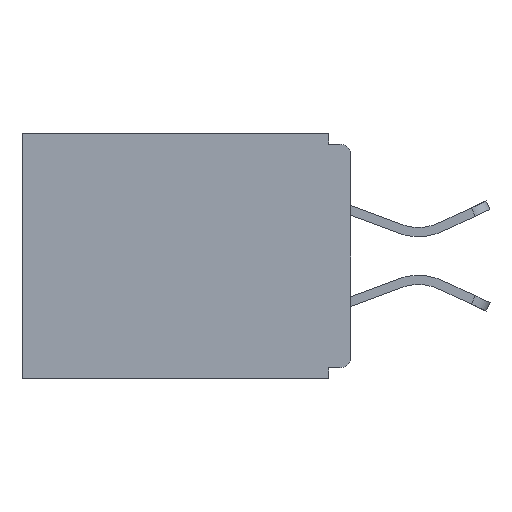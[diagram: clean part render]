
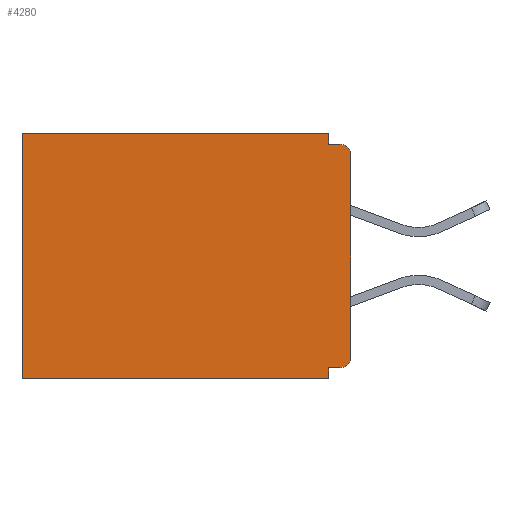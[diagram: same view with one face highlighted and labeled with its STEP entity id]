
A CAD part, left-side view. The second image highlights one B-rep face of the part: STEP entity #4280.
In plain terms, the highlighted planar face has unit normal (-1, 0, 0).
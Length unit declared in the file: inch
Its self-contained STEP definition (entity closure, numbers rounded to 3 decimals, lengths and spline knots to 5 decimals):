
#148 = DIRECTION ( 'NONE',  ( 0., 0., -1. ) ) ;
#595 = DIRECTION ( 'NONE',  ( -1., 0., 0. ) ) ;
#615 = PLANE ( 'NONE',  #6951 ) ;
#616 = VERTEX_POINT ( 'NONE', #11996 ) ;
#864 = VERTEX_POINT ( 'NONE', #12964 ) ;
#898 = CARTESIAN_POINT ( 'NONE',  ( 0.298, 0.031, -0.015 ) ) ;
#1536 = VERTEX_POINT ( 'NONE', #4678 ) ;
#1597 = EDGE_CURVE ( 'NONE', #10476, #2965, #2961, .T. ) ;
#1646 = CARTESIAN_POINT ( 'NONE',  ( 0.298, 0.031, -0.343 ) ) ;
#1675 = VERTEX_POINT ( 'NONE', #11287 ) ;
#1849 = CARTESIAN_POINT ( 'NONE',  ( 0.298, 0., 0. ) ) ;
#1911 = EDGE_CURVE ( 'NONE', #1536, #12967, #3587, .T. ) ;
#1960 = LINE ( 'NONE', #8977, #10019 ) ;
#1978 = VECTOR ( 'NONE', #6179, 39.37008 ) ;
#2581 = CARTESIAN_POINT ( 'NONE',  ( 0.298, 0.031, -0.343 ) ) ;
#2738 = CARTESIAN_POINT ( 'NONE',  ( 0.298, 0.015, -0.03 ) ) ;
#2759 = DIRECTION ( 'NONE',  ( 1., 0., 0. ) ) ;
#2955 = EDGE_CURVE ( 'NONE', #12348, #10156, #1960, .T. ) ;
#2961 = LINE ( 'NONE', #2581, #11042 ) ;
#2965 = VERTEX_POINT ( 'NONE', #1646 ) ;
#3064 = DIRECTION ( 'NONE',  ( 0., 1., 0. ) ) ;
#3109 = VECTOR ( 'NONE', #12346, 39.37008 ) ;
#3587 = LINE ( 'NONE', #12476, #8893 ) ;
#3760 = ORIENTED_EDGE ( 'NONE', *, *, #2955, .F. ) ;
#3929 = DIRECTION ( 'NONE',  ( 0., 0., -1. ) ) ;
#3978 = CARTESIAN_POINT ( 'NONE',  ( 0.298, 0.015, -0.015 ) ) ;
#4077 = ORIENTED_EDGE ( 'NONE', *, *, #9372, .T. ) ;
#4238 = ORIENTED_EDGE ( 'NONE', *, *, #1597, .F. ) ;
#4280 = ADVANCED_FACE ( 'NONE', ( #4674 ), #615, .F. ) ;
#4674 = FACE_OUTER_BOUND ( 'NONE', #10426, .T. ) ;
#4678 = CARTESIAN_POINT ( 'NONE',  ( 0.298, 0.031, 0. ) ) ;
#4708 = AXIS2_PLACEMENT_3D ( 'NONE', #8175, #6306, #9445 ) ;
#5553 = DIRECTION ( 'NONE',  ( 0., -1., 0. ) ) ;
#5603 = ORIENTED_EDGE ( 'NONE', *, *, #7041, .F. ) ;
#5711 = ORIENTED_EDGE ( 'NONE', *, *, #7684, .F. ) ;
#6006 = VERTEX_POINT ( 'NONE', #11267 ) ;
#6042 = ORIENTED_EDGE ( 'NONE', *, *, #1911, .T. ) ;
#6179 = DIRECTION ( 'NONE',  ( 0., 0., -1. ) ) ;
#6188 = DIRECTION ( 'NONE',  ( 0., 1., 0. ) ) ;
#6306 = DIRECTION ( 'NONE',  ( -1., 0., 0. ) ) ;
#6473 = ORIENTED_EDGE ( 'NONE', *, *, #11056, .T. ) ;
#6628 = VECTOR ( 'NONE', #8684, 39.37008 ) ;
#6683 = VECTOR ( 'NONE', #148, 39.37008 ) ;
#6951 = AXIS2_PLACEMENT_3D ( 'NONE', #1849, #2759, #3929 ) ;
#7041 = EDGE_CURVE ( 'NONE', #2965, #864, #10455, .T. ) ;
#7437 = CARTESIAN_POINT ( 'NONE',  ( 0.298, 0., 0. ) ) ;
#7562 = ORIENTED_EDGE ( 'NONE', *, *, #8576, .T. ) ;
#7569 = LINE ( 'NONE', #13562, #1978 ) ;
#7634 = VECTOR ( 'NONE', #3064, 39.37008 ) ;
#7684 = EDGE_CURVE ( 'NONE', #1675, #6006, #8781, .T. ) ;
#7711 = CARTESIAN_POINT ( 'NONE',  ( 0.298, 0.46, 0. ) ) ;
#7928 = DIRECTION ( 'NONE',  ( 0., 0., -1. ) ) ;
#7967 = AXIS2_PLACEMENT_3D ( 'NONE', #2738, #595, #7928 ) ;
#8098 = CARTESIAN_POINT ( 'NONE',  ( 0.298, 0., -0.328 ) ) ;
#8175 = CARTESIAN_POINT ( 'NONE',  ( 0.298, 0.015, -0.313 ) ) ;
#8576 = EDGE_CURVE ( 'NONE', #1675, #10156, #9905, .T. ) ;
#8684 = DIRECTION ( 'NONE',  ( 0., 0., -1. ) ) ;
#8781 = LINE ( 'NONE', #7437, #6628 ) ;
#8893 = VECTOR ( 'NONE', #6188, 39.37008 ) ;
#8977 = CARTESIAN_POINT ( 'NONE',  ( 0.298, 0., -0.015 ) ) ;
#9044 = EDGE_CURVE ( 'NONE', #616, #10476, #12858, .T. ) ;
#9372 = EDGE_CURVE ( 'NONE', #12967, #864, #7569, .T. ) ;
#9445 = DIRECTION ( 'NONE',  ( 0., 0., -1. ) ) ;
#9905 = CIRCLE ( 'NONE', #7967, 0.015 ) ;
#10019 = VECTOR ( 'NONE', #5553, 39.37008 ) ;
#10156 = VERTEX_POINT ( 'NONE', #3978 ) ;
#10426 = EDGE_LOOP ( 'NONE', ( #7562, #3760, #10877, #6042, #4077, #5603, #4238, #11911, #6473, #5711 ) ) ;
#10455 = LINE ( 'NONE', #11515, #7634 ) ;
#10476 = VERTEX_POINT ( 'NONE', #10955 ) ;
#10877 = ORIENTED_EDGE ( 'NONE', *, *, #11201, .F. ) ;
#10955 = CARTESIAN_POINT ( 'NONE',  ( 0.298, 0.031, -0.328 ) ) ;
#10969 = CIRCLE ( 'NONE', #4708, 0.015 ) ;
#11042 = VECTOR ( 'NONE', #12104, 39.37008 ) ;
#11056 = EDGE_CURVE ( 'NONE', #616, #6006, #10969, .T. ) ;
#11201 = EDGE_CURVE ( 'NONE', #1536, #12348, #12635, .T. ) ;
#11267 = CARTESIAN_POINT ( 'NONE',  ( 0.298, 0., -0.313 ) ) ;
#11287 = CARTESIAN_POINT ( 'NONE',  ( 0.298, 0., -0.03 ) ) ;
#11515 = CARTESIAN_POINT ( 'NONE',  ( 0.298, 0., -0.343 ) ) ;
#11846 = CARTESIAN_POINT ( 'NONE',  ( 0.298, 0.031, -0.343 ) ) ;
#11911 = ORIENTED_EDGE ( 'NONE', *, *, #9044, .F. ) ;
#11996 = CARTESIAN_POINT ( 'NONE',  ( 0.298, 0.015, -0.328 ) ) ;
#12104 = DIRECTION ( 'NONE',  ( 0., 0., -1. ) ) ;
#12346 = DIRECTION ( 'NONE',  ( 0., 1., 0. ) ) ;
#12348 = VERTEX_POINT ( 'NONE', #898 ) ;
#12476 = CARTESIAN_POINT ( 'NONE',  ( 0.298, 0., 0. ) ) ;
#12635 = LINE ( 'NONE', #11846, #6683 ) ;
#12858 = LINE ( 'NONE', #8098, #3109 ) ;
#12964 = CARTESIAN_POINT ( 'NONE',  ( 0.298, 0.46, -0.343 ) ) ;
#12967 = VERTEX_POINT ( 'NONE', #7711 ) ;
#13562 = CARTESIAN_POINT ( 'NONE',  ( 0.298, 0.46, 0. ) ) ;
